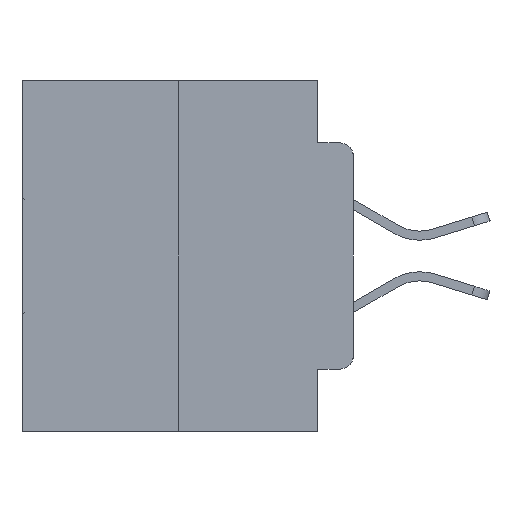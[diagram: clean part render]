
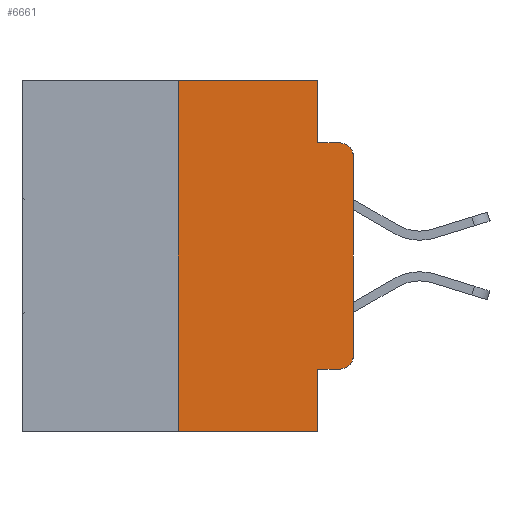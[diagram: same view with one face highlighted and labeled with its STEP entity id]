
A CAD part, left-side view. The second image highlights one B-rep face of the part: STEP entity #6661.
In plain terms, the highlighted planar face has unit normal (-1, 0, 0).
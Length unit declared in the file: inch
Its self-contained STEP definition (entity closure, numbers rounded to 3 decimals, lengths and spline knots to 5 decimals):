
#355 = LINE ( 'NONE', #9353, #29830 ) ;
#693 = VECTOR ( 'NONE', #2049, 39.37008 ) ;
#1732 = CARTESIAN_POINT ( 'NONE',  ( 0., 0.25, -0.5 ) ) ;
#2005 = ORIENTED_EDGE ( 'NONE', *, *, #17574, .F. ) ;
#2049 = DIRECTION ( 'NONE',  ( 0., -1., 0. ) ) ;
#2453 = EDGE_LOOP ( 'NONE', ( #11666, #11435, #2005, #17445, #11465, #10548, #5922, #6136, #14207, #16652 ) ) ;
#4964 = VECTOR ( 'NONE', #24249, 39.37008 ) ;
#5020 = EDGE_CURVE ( 'NONE', #10854, #20746, #23044, .T. ) ;
#5775 = CARTESIAN_POINT ( 'NONE',  ( 0., 0.473, 0. ) ) ;
#5922 = ORIENTED_EDGE ( 'NONE', *, *, #25645, .T. ) ;
#6136 = ORIENTED_EDGE ( 'NONE', *, *, #9868, .F. ) ;
#6661 = ADVANCED_FACE ( 'NONE', ( #14693 ), #10473, .F. ) ;
#6671 = EDGE_CURVE ( 'NONE', #29346, #10854, #15425, .T. ) ;
#7120 = VECTOR ( 'NONE', #12602, 39.37008 ) ;
#7402 = DIRECTION ( 'NONE',  ( -1., 0., 0. ) ) ;
#7610 = CARTESIAN_POINT ( 'NONE',  ( 0., 0.051, -0.4115 ) ) ;
#7734 = VERTEX_POINT ( 'NONE', #14663 ) ;
#8179 = DIRECTION ( 'NONE',  ( 0., 0., -1. ) ) ;
#8224 = CARTESIAN_POINT ( 'NONE',  ( 0., 0.02, -0.1085 ) ) ;
#8668 = LINE ( 'NONE', #14771, #15598 ) ;
#8824 = VECTOR ( 'NONE', #12091, 39.37008 ) ;
#9353 = CARTESIAN_POINT ( 'NONE',  ( 0., 0.051, 0. ) ) ;
#9358 = LINE ( 'NONE', #26336, #7120 ) ;
#9781 = CARTESIAN_POINT ( 'NONE',  ( 0., 0.051, 0. ) ) ;
#9868 = EDGE_CURVE ( 'NONE', #29346, #7734, #26458, .T. ) ;
#10473 = PLANE ( 'NONE',  #26614 ) ;
#10548 = ORIENTED_EDGE ( 'NONE', *, *, #11410, .F. ) ;
#10616 = DIRECTION ( 'NONE',  ( 0., 0., -1. ) ) ;
#10854 = VERTEX_POINT ( 'NONE', #26966 ) ;
#11410 = EDGE_CURVE ( 'NONE', #21944, #13045, #29521, .T. ) ;
#11435 = ORIENTED_EDGE ( 'NONE', *, *, #19116, .T. ) ;
#11465 = ORIENTED_EDGE ( 'NONE', *, *, #16688, .F. ) ;
#11666 = ORIENTED_EDGE ( 'NONE', *, *, #26765, .T. ) ;
#12091 = DIRECTION ( 'NONE',  ( 0., 0., -1. ) ) ;
#12401 = VERTEX_POINT ( 'NONE', #19731 ) ;
#12602 = DIRECTION ( 'NONE',  ( 0., -1., 0. ) ) ;
#13045 = VERTEX_POINT ( 'NONE', #15208 ) ;
#13866 = CARTESIAN_POINT ( 'NONE',  ( 0., 0.473, 0. ) ) ;
#14207 = ORIENTED_EDGE ( 'NONE', *, *, #6671, .T. ) ;
#14583 = LINE ( 'NONE', #24445, #25325 ) ;
#14663 = CARTESIAN_POINT ( 'NONE',  ( 0., 0.051, -0.5 ) ) ;
#14693 = FACE_OUTER_BOUND ( 'NONE', #2453, .T. ) ;
#14771 = CARTESIAN_POINT ( 'NONE',  ( 0., 0., 0. ) ) ;
#15057 = CARTESIAN_POINT ( 'NONE',  ( 0., 0.25, 0. ) ) ;
#15208 = CARTESIAN_POINT ( 'NONE',  ( 0., 0.25, 0. ) ) ;
#15219 = DIRECTION ( 'NONE',  ( 0., -1., 0. ) ) ;
#15425 = LINE ( 'NONE', #24305, #20770 ) ;
#15598 = VECTOR ( 'NONE', #28414, 39.37008 ) ;
#15945 = AXIS2_PLACEMENT_3D ( 'NONE', #8224, #24352, #10616 ) ;
#16056 = EDGE_CURVE ( 'NONE', #12401, #23264, #355, .T. ) ;
#16652 = ORIENTED_EDGE ( 'NONE', *, *, #5020, .T. ) ;
#16688 = EDGE_CURVE ( 'NONE', #13045, #12401, #20201, .T. ) ;
#17011 = VERTEX_POINT ( 'NONE', #24074 ) ;
#17445 = ORIENTED_EDGE ( 'NONE', *, *, #16056, .F. ) ;
#17574 = EDGE_CURVE ( 'NONE', #23264, #17011, #9358, .T. ) ;
#19116 = EDGE_CURVE ( 'NONE', #21911, #17011, #21841, .T. ) ;
#19731 = CARTESIAN_POINT ( 'NONE',  ( 0., 0.051, 0. ) ) ;
#20201 = LINE ( 'NONE', #13866, #693 ) ;
#20746 = VERTEX_POINT ( 'NONE', #23573 ) ;
#20770 = VECTOR ( 'NONE', #15219, 39.37008 ) ;
#20925 = DIRECTION ( 'NONE',  ( 0., 0., -1. ) ) ;
#21247 = CARTESIAN_POINT ( 'NONE',  ( 0., 0.02, -0.3915 ) ) ;
#21841 = CIRCLE ( 'NONE', #15945, 0.02 ) ;
#21911 = VERTEX_POINT ( 'NONE', #27182 ) ;
#21944 = VERTEX_POINT ( 'NONE', #1732 ) ;
#21996 = DIRECTION ( 'NONE',  ( 1., 0., 0. ) ) ;
#22362 = AXIS2_PLACEMENT_3D ( 'NONE', #21247, #7402, #23548 ) ;
#23044 = CIRCLE ( 'NONE', #22362, 0.02 ) ;
#23049 = CARTESIAN_POINT ( 'NONE',  ( 0., 0.051, -0.0885 ) ) ;
#23264 = VERTEX_POINT ( 'NONE', #23049 ) ;
#23548 = DIRECTION ( 'NONE',  ( 0., 0., -1. ) ) ;
#23573 = CARTESIAN_POINT ( 'NONE',  ( 0., 0., -0.3915 ) ) ;
#24074 = CARTESIAN_POINT ( 'NONE',  ( 0., 0.02, -0.0885 ) ) ;
#24249 = DIRECTION ( 'NONE',  ( 0., 0., 1. ) ) ;
#24305 = CARTESIAN_POINT ( 'NONE',  ( 0., 0.051, -0.4115 ) ) ;
#24352 = DIRECTION ( 'NONE',  ( -1., 0., 0. ) ) ;
#24445 = CARTESIAN_POINT ( 'NONE',  ( 0., 0.473, -0.5 ) ) ;
#25325 = VECTOR ( 'NONE', #26723, 39.37008 ) ;
#25645 = EDGE_CURVE ( 'NONE', #21944, #7734, #14583, .T. ) ;
#26336 = CARTESIAN_POINT ( 'NONE',  ( 0., 0.051, -0.0885 ) ) ;
#26458 = LINE ( 'NONE', #9781, #8824 ) ;
#26614 = AXIS2_PLACEMENT_3D ( 'NONE', #5775, #21996, #8179 ) ;
#26723 = DIRECTION ( 'NONE',  ( 0., -1., 0. ) ) ;
#26765 = EDGE_CURVE ( 'NONE', #20746, #21911, #8668, .T. ) ;
#26966 = CARTESIAN_POINT ( 'NONE',  ( 0., 0.02, -0.4115 ) ) ;
#27182 = CARTESIAN_POINT ( 'NONE',  ( 0., 0., -0.1085 ) ) ;
#28414 = DIRECTION ( 'NONE',  ( 0., 0., 1. ) ) ;
#29346 = VERTEX_POINT ( 'NONE', #7610 ) ;
#29521 = LINE ( 'NONE', #15057, #4964 ) ;
#29830 = VECTOR ( 'NONE', #20925, 39.37008 ) ;
